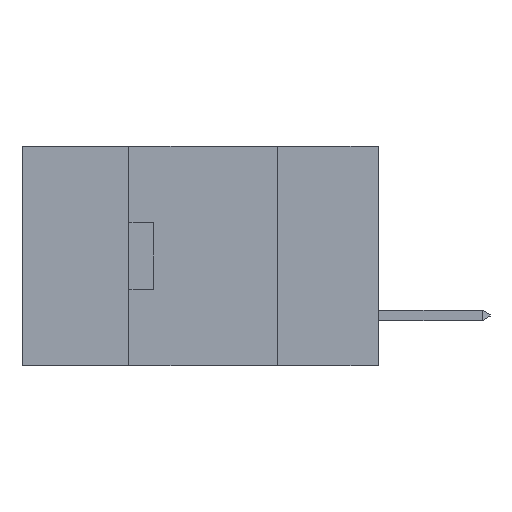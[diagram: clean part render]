
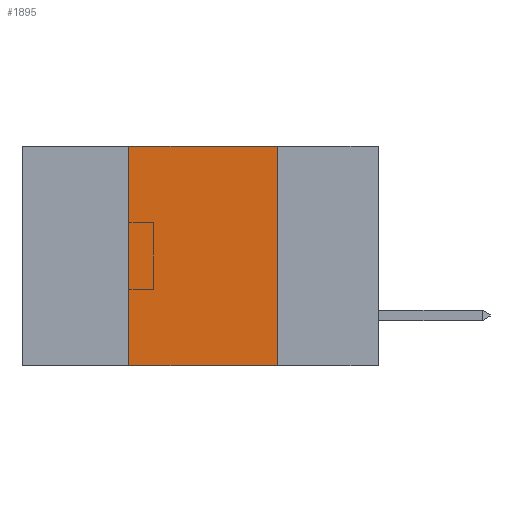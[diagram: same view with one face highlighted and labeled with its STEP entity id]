
A CAD part, left-side view. The second image highlights one B-rep face of the part: STEP entity #1895.
In plain terms, the highlighted planar face has unit normal (-1, 0, 0).
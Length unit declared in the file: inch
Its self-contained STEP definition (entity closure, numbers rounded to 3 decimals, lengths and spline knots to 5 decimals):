
#123 = CARTESIAN_POINT ( 'NONE',  ( 0., 0.42, -0.37 ) ) ;
#496 = EDGE_CURVE ( 'NONE', #8560, #2363, #15044, .T. ) ;
#1895 = ADVANCED_FACE ( 'NONE', ( #18504 ), #25587, .F. ) ;
#2351 = LINE ( 'NONE', #6206, #18477 ) ;
#2363 = VERTEX_POINT ( 'NONE', #22030 ) ;
#3250 = ORIENTED_EDGE ( 'NONE', *, *, #20778, .F. ) ;
#3323 = AXIS2_PLACEMENT_3D ( 'NONE', #24356, #23796, #23362 ) ;
#4619 = DIRECTION ( 'NONE',  ( 0., -1., 0. ) ) ;
#5391 = CARTESIAN_POINT ( 'NONE',  ( 0., 0.42, -0.37 ) ) ;
#5957 = DIRECTION ( 'NONE',  ( 0., 0., -1. ) ) ;
#6206 = CARTESIAN_POINT ( 'NONE',  ( 0., 0.6, -0.37 ) ) ;
#8043 = EDGE_CURVE ( 'NONE', #11380, #24490, #2351, .T. ) ;
#8560 = VERTEX_POINT ( 'NONE', #17260 ) ;
#9402 = VECTOR ( 'NONE', #24298, 39.37008 ) ;
#11380 = VERTEX_POINT ( 'NONE', #5391 ) ;
#11553 = EDGE_CURVE ( 'NONE', #2363, #24490, #18057, .T. ) ;
#12537 = VECTOR ( 'NONE', #5957, 39.37008 ) ;
#12600 = EDGE_LOOP ( 'NONE', ( #26098, #21605, #3250, #21576 ) ) ;
#13172 = CARTESIAN_POINT ( 'NONE',  ( 0., 0.17, -0.37 ) ) ;
#14976 = VECTOR ( 'NONE', #15016, 39.37008 ) ;
#15016 = DIRECTION ( 'NONE',  ( 0., 0., 1. ) ) ;
#15044 = LINE ( 'NONE', #23734, #9402 ) ;
#17260 = CARTESIAN_POINT ( 'NONE',  ( 0., 0.42, 0. ) ) ;
#18057 = LINE ( 'NONE', #22616, #12537 ) ;
#18477 = VECTOR ( 'NONE', #4619, 39.37008 ) ;
#18504 = FACE_OUTER_BOUND ( 'NONE', #12600, .T. ) ;
#20438 = LINE ( 'NONE', #123, #14976 ) ;
#20778 = EDGE_CURVE ( 'NONE', #11380, #8560, #20438, .T. ) ;
#21576 = ORIENTED_EDGE ( 'NONE', *, *, #8043, .T. ) ;
#21605 = ORIENTED_EDGE ( 'NONE', *, *, #496, .F. ) ;
#22030 = CARTESIAN_POINT ( 'NONE',  ( 0., 0.17, 0. ) ) ;
#22616 = CARTESIAN_POINT ( 'NONE',  ( 0., 0.17, -0.37 ) ) ;
#23362 = DIRECTION ( 'NONE',  ( 0., 0., -1. ) ) ;
#23734 = CARTESIAN_POINT ( 'NONE',  ( 0., 0.6, 0. ) ) ;
#23796 = DIRECTION ( 'NONE',  ( 1., 0., 0. ) ) ;
#24298 = DIRECTION ( 'NONE',  ( 0., -1., 0. ) ) ;
#24356 = CARTESIAN_POINT ( 'NONE',  ( 0., 0.6, 0. ) ) ;
#24490 = VERTEX_POINT ( 'NONE', #13172 ) ;
#25587 = PLANE ( 'NONE',  #3323 ) ;
#26098 = ORIENTED_EDGE ( 'NONE', *, *, #11553, .F. ) ;
